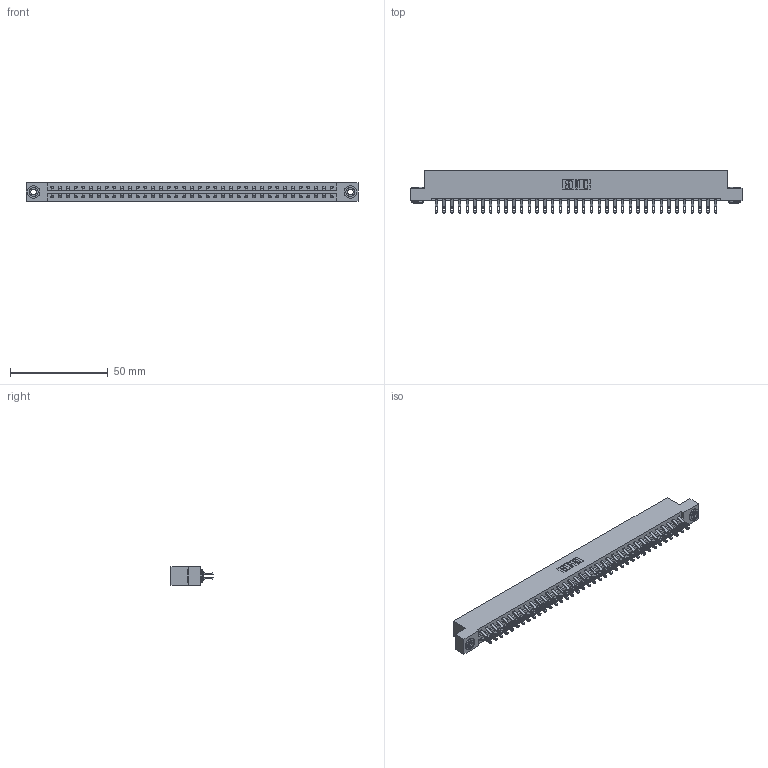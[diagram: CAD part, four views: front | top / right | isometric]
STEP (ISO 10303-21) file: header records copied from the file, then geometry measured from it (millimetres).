
FILE_DESCRIPTION (( 'STEP AP203' ), '1' );
FILE_NAME ('337-074-555-203.STEP', '2019-10-10T04:05:26', ( '' ), ( '' ), 'SwSTEP 2.0', 'SolidWorks 2016', '' );
FILE_SCHEMA (( 'CONFIG_CONTROL_DESIGN' ));
Length unit declared in the file: inch
Products named in the file (4): 337-074-555-203; 345-292-001_555 Tail; 345-250-002_345-250-002-102; 337 Part_Flush Mounting Lugs - 0.156 Dia-TH
Assembly tree (77 placements, depth 2):
  337-074-555-203
    337 Part_Flush Mounting Lugs - 0.156 Dia-TH
    345-292-001_555 Tail  x74
    345-250-002_345-250-002-102  x2
Bounding box: 169.62 x 21.47 x 9.4 mm (x, y, z)
Volume: 18043.5 mm3; surface area: 21382.9 mm2
Topology: 77 solids, 77 shells, 4592 faces, 14373 edges, 9578 vertices
Faces by surface type: plane 2744, cylinder 1840, cone 8
Entity records: 30310 total; most frequent: CARTESIAN_POINT 5119, ORIENTED_EDGE 5018, DIRECTION 4367, EDGE_CURVE 2509, LINE 2337, VECTOR 2337, VERTEX_POINT 1670, AXIS2_PLACEMENT_3D 1015
